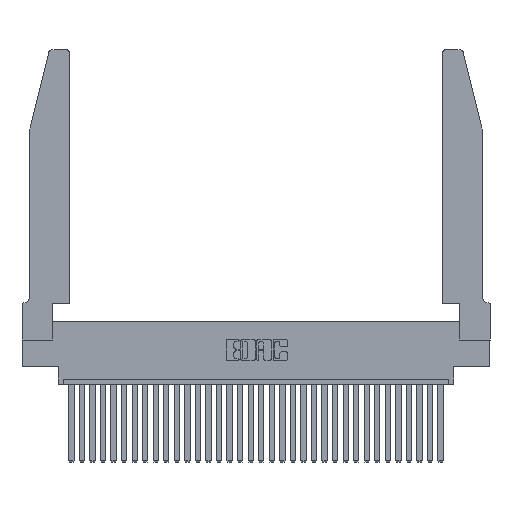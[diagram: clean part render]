
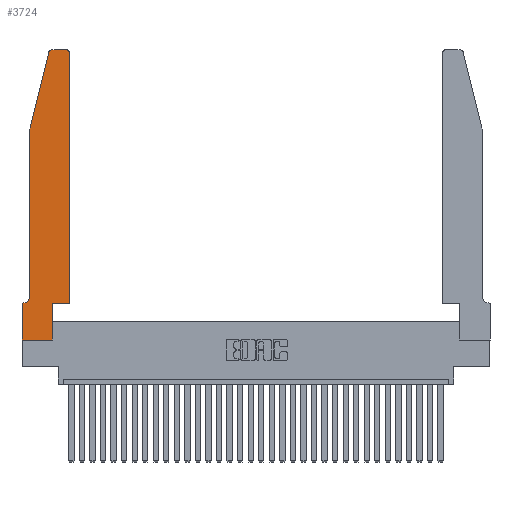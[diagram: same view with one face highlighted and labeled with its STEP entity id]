
A CAD part, top view. The second image highlights one B-rep face of the part: STEP entity #3724.
In plain terms, the highlighted planar face has unit normal (0, 0, 1).
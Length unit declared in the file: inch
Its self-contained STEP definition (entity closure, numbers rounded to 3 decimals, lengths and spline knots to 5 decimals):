
#164 = LINE ( 'NONE', #20743, #28122 ) ;
#974 = CARTESIAN_POINT ( 'NONE',  ( 0.4505, 0.35, 0.37 ) ) ;
#996 = AXIS2_PLACEMENT_3D ( 'NONE', #2364, #24644, #19705 ) ;
#1299 = VECTOR ( 'NONE', #29478, 39.37008 ) ;
#1630 = CARTESIAN_POINT ( 'NONE',  ( 0.4205, 2.72, 0.37 ) ) ;
#1799 = LINE ( 'NONE', #18187, #18391 ) ;
#2172 = EDGE_CURVE ( 'NONE', #11844, #14898, #19444, .T. ) ;
#2180 = CARTESIAN_POINT ( 'NONE',  ( 0.2605, 2.75, 0.37 ) ) ;
#2364 = CARTESIAN_POINT ( 'NONE',  ( 0.284, 2.72, 0.37 ) ) ;
#2375 = CARTESIAN_POINT ( 'NONE',  ( 0., 0., 0.37 ) ) ;
#2409 = LINE ( 'NONE', #21905, #7561 ) ;
#2469 = AXIS2_PLACEMENT_3D ( 'NONE', #9457, #22108, #31817 ) ;
#2823 = DIRECTION ( 'NONE',  ( 0., 1., 0. ) ) ;
#3264 = CARTESIAN_POINT ( 'NONE',  ( 0.2865, 0., 0.37 ) ) ;
#3598 = CIRCLE ( 'NONE', #12164, 0.07 ) ;
#3616 = CARTESIAN_POINT ( 'NONE',  ( 0.0755, 2., 0.37 ) ) ;
#3724 = ADVANCED_FACE ( 'NONE', ( #20104 ), #14619, .T. ) ;
#3738 = EDGE_CURVE ( 'NONE', #14214, #13027, #15735, .T. ) ;
#3804 = VERTEX_POINT ( 'NONE', #22665 ) ;
#4483 = VERTEX_POINT ( 'NONE', #25657 ) ;
#5290 = VERTEX_POINT ( 'NONE', #19623 ) ;
#5491 = EDGE_CURVE ( 'NONE', #5565, #14214, #30235, .T. ) ;
#5565 = VERTEX_POINT ( 'NONE', #974 ) ;
#6813 = DIRECTION ( 'NONE',  ( -0.239, -0.971, 0. ) ) ;
#7363 = ORIENTED_EDGE ( 'NONE', *, *, #19014, .T. ) ;
#7561 = VECTOR ( 'NONE', #6813, 39.37008 ) ;
#8222 = ORIENTED_EDGE ( 'NONE', *, *, #21411, .T. ) ;
#8445 = VECTOR ( 'NONE', #9691, 39.37008 ) ;
#8579 = ORIENTED_EDGE ( 'NONE', *, *, #20158, .T. ) ;
#8653 = CARTESIAN_POINT ( 'NONE',  ( 0.0755, 2., 0.37 ) ) ;
#8806 = ORIENTED_EDGE ( 'NONE', *, *, #17202, .T. ) ;
#8980 = ORIENTED_EDGE ( 'NONE', *, *, #13709, .T. ) ;
#9245 = ORIENTED_EDGE ( 'NONE', *, *, #5491, .T. ) ;
#9457 = CARTESIAN_POINT ( 'NONE',  ( 0., 0.35, 0.37 ) ) ;
#9655 = LINE ( 'NONE', #2180, #8445 ) ;
#9691 = DIRECTION ( 'NONE',  ( -1., 0., 0. ) ) ;
#9750 = VERTEX_POINT ( 'NONE', #8653 ) ;
#10307 = AXIS2_PLACEMENT_3D ( 'NONE', #1630, #16613, #29362 ) ;
#10385 = DIRECTION ( 'NONE',  ( -1., 0., 0. ) ) ;
#10710 = DIRECTION ( 'NONE',  ( 0., 1., 0. ) ) ;
#11233 = LINE ( 'NONE', #24647, #28130 ) ;
#11844 = VERTEX_POINT ( 'NONE', #21930 ) ;
#12164 = AXIS2_PLACEMENT_3D ( 'NONE', #15517, #23020, #20290 ) ;
#13027 = VERTEX_POINT ( 'NONE', #26578 ) ;
#13183 = VERTEX_POINT ( 'NONE', #18956 ) ;
#13709 = EDGE_CURVE ( 'NONE', #9750, #21278, #25205, .T. ) ;
#14214 = VERTEX_POINT ( 'NONE', #19182 ) ;
#14402 = VECTOR ( 'NONE', #10385, 39.37008 ) ;
#14501 = DIRECTION ( 'NONE',  ( 0., -1., 0. ) ) ;
#14619 = PLANE ( 'NONE',  #2469 ) ;
#14898 = VERTEX_POINT ( 'NONE', #3264 ) ;
#15253 = ORIENTED_EDGE ( 'NONE', *, *, #18720, .T. ) ;
#15517 = CARTESIAN_POINT ( 'NONE',  ( 0.0055, 0.42, 0.37 ) ) ;
#15735 = CIRCLE ( 'NONE', #10307, 0.03 ) ;
#16559 = EDGE_CURVE ( 'NONE', #13183, #3804, #27017, .T. ) ;
#16613 = DIRECTION ( 'NONE',  ( 0., 0., 1. ) ) ;
#17202 = EDGE_CURVE ( 'NONE', #14898, #4483, #164, .T. ) ;
#17556 = CARTESIAN_POINT ( 'NONE',  ( 0.25487, 2.72718, 0.37 ) ) ;
#18187 = CARTESIAN_POINT ( 'NONE',  ( 0.4505, 0.35, 0.37 ) ) ;
#18391 = VECTOR ( 'NONE', #25979, 39.37008 ) ;
#18720 = EDGE_CURVE ( 'NONE', #21278, #13183, #3598, .T. ) ;
#18956 = CARTESIAN_POINT ( 'NONE',  ( 0.0055, 0.35, 0.37 ) ) ;
#19014 = EDGE_CURVE ( 'NONE', #26575, #9750, #2409, .T. ) ;
#19182 = CARTESIAN_POINT ( 'NONE',  ( 0.4505, 2.72, 0.37 ) ) ;
#19444 = LINE ( 'NONE', #2375, #1299 ) ;
#19623 = CARTESIAN_POINT ( 'NONE',  ( 0.284, 2.75, 0.37 ) ) ;
#19705 = DIRECTION ( 'NONE',  ( 1., 0., 0. ) ) ;
#19918 = EDGE_CURVE ( 'NONE', #4483, #5565, #1799, .T. ) ;
#20104 = FACE_OUTER_BOUND ( 'NONE', #25850, .T. ) ;
#20158 = EDGE_CURVE ( 'NONE', #5290, #26575, #30944, .T. ) ;
#20290 = DIRECTION ( 'NONE',  ( -1., 0., 0. ) ) ;
#20743 = CARTESIAN_POINT ( 'NONE',  ( 0.2865, 0.35, 0.37 ) ) ;
#20864 = ORIENTED_EDGE ( 'NONE', *, *, #3738, .T. ) ;
#21278 = VERTEX_POINT ( 'NONE', #24000 ) ;
#21411 = EDGE_CURVE ( 'NONE', #3804, #11844, #11233, .T. ) ;
#21905 = CARTESIAN_POINT ( 'NONE',  ( 0.0755, 2., 0.37 ) ) ;
#21930 = CARTESIAN_POINT ( 'NONE',  ( 0., 0., 0.37 ) ) ;
#22108 = DIRECTION ( 'NONE',  ( 0., 0., 1. ) ) ;
#22568 = ORIENTED_EDGE ( 'NONE', *, *, #2172, .T. ) ;
#22665 = CARTESIAN_POINT ( 'NONE',  ( 0., 0.35, 0.37 ) ) ;
#22704 = CARTESIAN_POINT ( 'NONE',  ( 0.4505, 0.35, 0.37 ) ) ;
#22841 = CARTESIAN_POINT ( 'NONE',  ( 0.0755, 0.35, 0.37 ) ) ;
#23020 = DIRECTION ( 'NONE',  ( 0., 0., -1. ) ) ;
#23147 = ORIENTED_EDGE ( 'NONE', *, *, #29962, .T. ) ;
#23199 = ORIENTED_EDGE ( 'NONE', *, *, #19918, .T. ) ;
#24000 = CARTESIAN_POINT ( 'NONE',  ( 0.0755, 0.42, 0.37 ) ) ;
#24425 = VECTOR ( 'NONE', #32471, 39.37008 ) ;
#24644 = DIRECTION ( 'NONE',  ( 0., 0., 1. ) ) ;
#24647 = CARTESIAN_POINT ( 'NONE',  ( 0., 0., 0.37 ) ) ;
#25205 = LINE ( 'NONE', #3616, #24425 ) ;
#25657 = CARTESIAN_POINT ( 'NONE',  ( 0.2865, 0.35, 0.37 ) ) ;
#25850 = EDGE_LOOP ( 'NONE', ( #23147, #8579, #7363, #8980, #15253, #32225, #8222, #22568, #8806, #23199, #9245, #20864 ) ) ;
#25979 = DIRECTION ( 'NONE',  ( 1., 0., 0. ) ) ;
#26575 = VERTEX_POINT ( 'NONE', #17556 ) ;
#26578 = CARTESIAN_POINT ( 'NONE',  ( 0.4205, 2.75, 0.37 ) ) ;
#27017 = LINE ( 'NONE', #22841, #14402 ) ;
#28122 = VECTOR ( 'NONE', #10710, 39.37008 ) ;
#28130 = VECTOR ( 'NONE', #14501, 39.37008 ) ;
#29362 = DIRECTION ( 'NONE',  ( 1., 0., 0. ) ) ;
#29478 = DIRECTION ( 'NONE',  ( 1., 0., 0. ) ) ;
#29962 = EDGE_CURVE ( 'NONE', #13027, #5290, #9655, .T. ) ;
#30235 = LINE ( 'NONE', #22704, #31046 ) ;
#30944 = CIRCLE ( 'NONE', #996, 0.03 ) ;
#31046 = VECTOR ( 'NONE', #2823, 39.37008 ) ;
#31817 = DIRECTION ( 'NONE',  ( 1., 0., 0. ) ) ;
#32225 = ORIENTED_EDGE ( 'NONE', *, *, #16559, .T. ) ;
#32471 = DIRECTION ( 'NONE',  ( 0., -1., 0. ) ) ;
